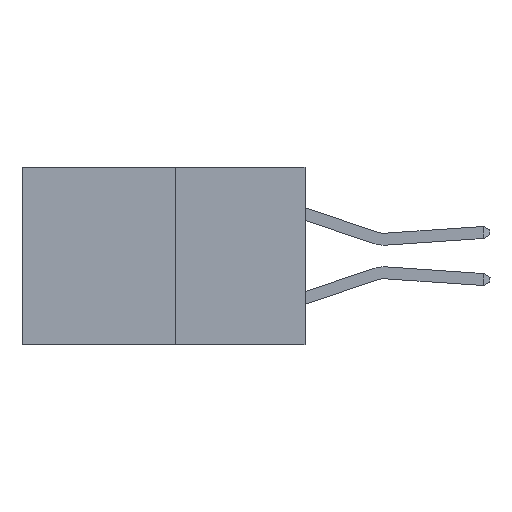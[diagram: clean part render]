
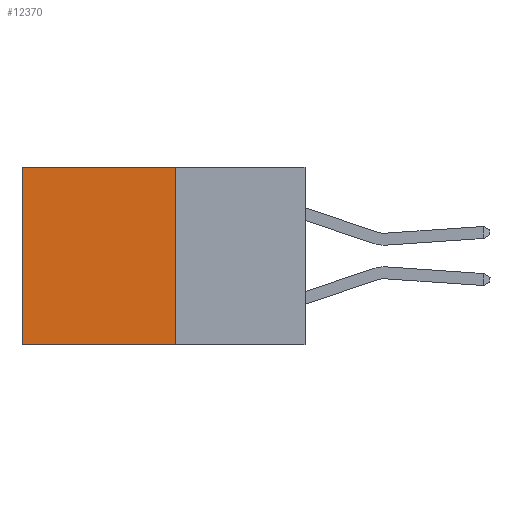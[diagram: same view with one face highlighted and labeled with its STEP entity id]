
A CAD part, left-side view. The second image highlights one B-rep face of the part: STEP entity #12370.
In plain terms, the highlighted planar face has unit normal (-1, 0, 0).
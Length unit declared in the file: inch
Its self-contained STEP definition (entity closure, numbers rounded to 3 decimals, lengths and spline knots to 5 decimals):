
#269 = VERTEX_POINT ( 'NONE', #9288 ) ;
#339 = CARTESIAN_POINT ( 'NONE',  ( 0.277, 0.59, -0.37 ) ) ;
#1108 = VECTOR ( 'NONE', #9839, 39.37008 ) ;
#1362 = VERTEX_POINT ( 'NONE', #22273 ) ;
#1449 = AXIS2_PLACEMENT_3D ( 'NONE', #14071, #23207, #12303 ) ;
#4333 = DIRECTION ( 'NONE',  ( 0., 1., 0. ) ) ;
#4567 = EDGE_LOOP ( 'NONE', ( #22034, #20643, #4579, #15320 ) ) ;
#4568 = CARTESIAN_POINT ( 'NONE',  ( 0.277, 0.27, -0.37 ) ) ;
#4579 = ORIENTED_EDGE ( 'NONE', *, *, #21111, .F. ) ;
#4845 = EDGE_CURVE ( 'NONE', #1362, #14922, #5738, .T. ) ;
#5613 = LINE ( 'NONE', #7907, #1108 ) ;
#5738 = LINE ( 'NONE', #4568, #15118 ) ;
#6595 = PLANE ( 'NONE',  #1449 ) ;
#7220 = LINE ( 'NONE', #15349, #15955 ) ;
#7907 = CARTESIAN_POINT ( 'NONE',  ( 0.277, 0.59, -0.37 ) ) ;
#9288 = CARTESIAN_POINT ( 'NONE',  ( 0.277, 0.59, 0. ) ) ;
#9839 = DIRECTION ( 'NONE',  ( 0., 0., -1. ) ) ;
#10832 = CARTESIAN_POINT ( 'NONE',  ( 0.277, 0.27, 0. ) ) ;
#11339 = LINE ( 'NONE', #17673, #20505 ) ;
#11761 = EDGE_CURVE ( 'NONE', #12527, #269, #11339, .T. ) ;
#12303 = DIRECTION ( 'NONE',  ( 0., 0., -1. ) ) ;
#12370 = ADVANCED_FACE ( 'NONE', ( #13909 ), #6595, .F. ) ;
#12527 = VERTEX_POINT ( 'NONE', #10832 ) ;
#13546 = EDGE_CURVE ( 'NONE', #269, #14922, #5613, .T. ) ;
#13909 = FACE_OUTER_BOUND ( 'NONE', #4567, .T. ) ;
#14071 = CARTESIAN_POINT ( 'NONE',  ( 0.277, 0.27, -0.37 ) ) ;
#14922 = VERTEX_POINT ( 'NONE', #339 ) ;
#15118 = VECTOR ( 'NONE', #4333, 39.37008 ) ;
#15320 = ORIENTED_EDGE ( 'NONE', *, *, #11761, .T. ) ;
#15349 = CARTESIAN_POINT ( 'NONE',  ( 0.277, 0.27, -0.37 ) ) ;
#15955 = VECTOR ( 'NONE', #17158, 39.37008 ) ;
#17158 = DIRECTION ( 'NONE',  ( 0., 0., -1. ) ) ;
#17673 = CARTESIAN_POINT ( 'NONE',  ( 0.277, 0.27, 0. ) ) ;
#19524 = DIRECTION ( 'NONE',  ( 0., 1., 0. ) ) ;
#20505 = VECTOR ( 'NONE', #19524, 39.37008 ) ;
#20643 = ORIENTED_EDGE ( 'NONE', *, *, #4845, .F. ) ;
#21111 = EDGE_CURVE ( 'NONE', #12527, #1362, #7220, .T. ) ;
#22034 = ORIENTED_EDGE ( 'NONE', *, *, #13546, .T. ) ;
#22273 = CARTESIAN_POINT ( 'NONE',  ( 0.277, 0.27, -0.37 ) ) ;
#23207 = DIRECTION ( 'NONE',  ( 1., 0., 0. ) ) ;
